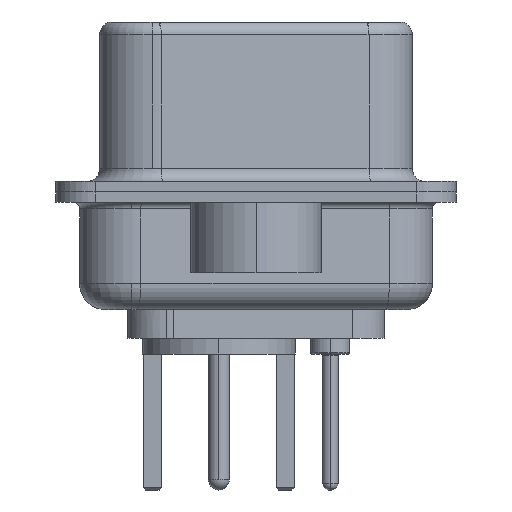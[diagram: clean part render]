
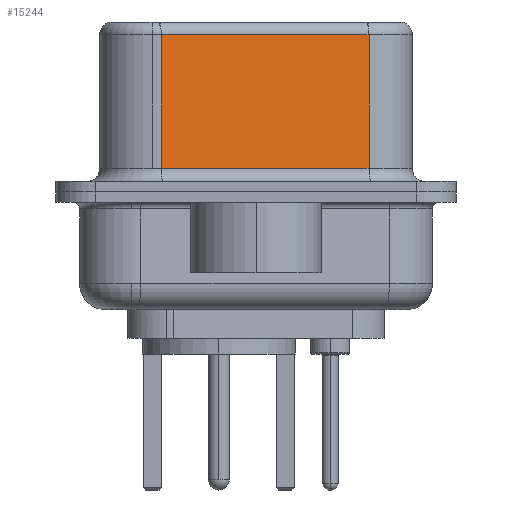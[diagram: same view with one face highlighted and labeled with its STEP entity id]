
A CAD part, left-side view. The second image highlights one B-rep face of the part: STEP entity #15244.
In plain terms, the highlighted planar face has unit normal (-0.985, -0.174, 0).
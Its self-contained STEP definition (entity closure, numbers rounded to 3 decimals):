
#180 = AXIS2_PLACEMENT_3D ( 'NONE', #16398, #10800, #23932 ) ;
#2820 = CARTESIAN_POINT ( 'NONE',  ( 5.132, -4.322, 6.52 ) ) ;
#3052 = LINE ( 'NONE', #7704, #16640 ) ;
#3287 = CARTESIAN_POINT ( 'NONE',  ( 5.132, -4.322, 6.02 ) ) ;
#4347 = DIRECTION ( 'NONE',  ( 0.174, -0.985, 0. ) ) ;
#4780 = ORIENTED_EDGE ( 'NONE', *, *, #15452, .T. ) ;
#4991 = LINE ( 'NONE', #8042, #23649 ) ;
#5345 = VERTEX_POINT ( 'NONE', #23348 ) ;
#5453 = VERTEX_POINT ( 'NONE', #14216 ) ;
#5836 = DIRECTION ( 'NONE',  ( 0., 0., -1. ) ) ;
#6596 = DIRECTION ( 'NONE',  ( 0., 0., -1. ) ) ;
#7421 = VERTEX_POINT ( 'NONE', #12019 ) ;
#7704 = CARTESIAN_POINT ( 'NONE',  ( 3.73, 3.628, 6.52 ) ) ;
#8042 = CARTESIAN_POINT ( 'NONE',  ( 5.132, -4.322, 0.9 ) ) ;
#8363 = EDGE_LOOP ( 'NONE', ( #13789, #19641, #4780, #12136 ) ) ;
#10800 = DIRECTION ( 'NONE',  ( 0.985, 0.174, 0. ) ) ;
#11528 = CARTESIAN_POINT ( 'NONE',  ( 5.132, -4.322, 6.02 ) ) ;
#12019 = CARTESIAN_POINT ( 'NONE',  ( 5.132, -4.322, 0.9 ) ) ;
#12136 = ORIENTED_EDGE ( 'NONE', *, *, #21898, .T. ) ;
#12475 = DIRECTION ( 'NONE',  ( -0.174, 0.985, 0. ) ) ;
#13092 = VECTOR ( 'NONE', #12475, 1000. ) ;
#13710 = LINE ( 'NONE', #3287, #13092 ) ;
#13789 = ORIENTED_EDGE ( 'NONE', *, *, #16239, .F. ) ;
#14216 = CARTESIAN_POINT ( 'NONE',  ( 3.73, 3.628, 6.02 ) ) ;
#15244 = ADVANCED_FACE ( 'NONE', ( #20154 ), #21949, .F. ) ;
#15452 = EDGE_CURVE ( 'NONE', #5453, #5345, #3052, .T. ) ;
#16239 = EDGE_CURVE ( 'NONE', #19973, #7421, #23095, .T. ) ;
#16398 = CARTESIAN_POINT ( 'NONE',  ( 5.132, -4.322, 6.52 ) ) ;
#16640 = VECTOR ( 'NONE', #5836, 1000. ) ;
#18097 = VECTOR ( 'NONE', #6596, 1000. ) ;
#19641 = ORIENTED_EDGE ( 'NONE', *, *, #20347, .T. ) ;
#19973 = VERTEX_POINT ( 'NONE', #11528 ) ;
#20154 = FACE_OUTER_BOUND ( 'NONE', #8363, .T. ) ;
#20347 = EDGE_CURVE ( 'NONE', #19973, #5453, #13710, .T. ) ;
#21898 = EDGE_CURVE ( 'NONE', #5345, #7421, #4991, .T. ) ;
#21949 = PLANE ( 'NONE',  #180 ) ;
#23095 = LINE ( 'NONE', #2820, #18097 ) ;
#23348 = CARTESIAN_POINT ( 'NONE',  ( 3.73, 3.628, 0.9 ) ) ;
#23649 = VECTOR ( 'NONE', #4347, 1000. ) ;
#23932 = DIRECTION ( 'NONE',  ( -0.174, 0.985, 0. ) ) ;
